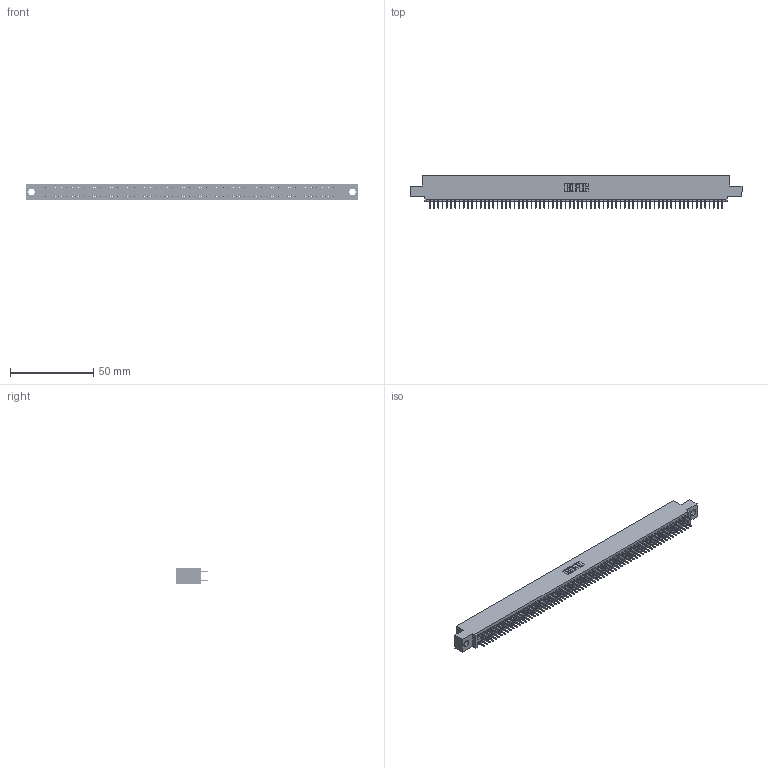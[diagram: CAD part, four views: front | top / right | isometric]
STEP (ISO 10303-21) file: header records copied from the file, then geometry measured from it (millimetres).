
FILE_DESCRIPTION (( 'STEP AP203' ), '1' );
FILE_NAME ('395-140-524-504.STEP', '2021-06-18T04:21:42', ( '' ), ( '' ), 'SwSTEP 2.0', 'SolidWorks 2020', '' );
FILE_SCHEMA (( 'CONFIG_CONTROL_DESIGN' ));
Length unit declared in the file: inch
Products named in the file (3): 345 Part_0.110 Offset - 0.156 Dia-TI; 395-140-524-504; 345-292-001_345-293-124
Assembly tree (141 placements, depth 2):
  395-140-524-504
    345 Part_0.110 Offset - 0.156 Dia-TI
    345-292-001_345-293-124  x140
Bounding box: 199.01 x 19.35 x 9.4 mm (x, y, z)
Volume: 19200.7 mm3; surface area: 28309.2 mm2
Topology: 141 solids, 141 shells, 7704 faces, 21809 edges, 13978 vertices
Faces by surface type: plane 5558, cylinder 2146
Entity records: 51779 total; most frequent: CARTESIAN_POINT 8658, ORIENTED_EDGE 8590, DIRECTION 7599, EDGE_CURVE 4295, LINE 3887, VECTOR 3887, VERTEX_POINT 2858, AXIS2_PLACEMENT_3D 1856
